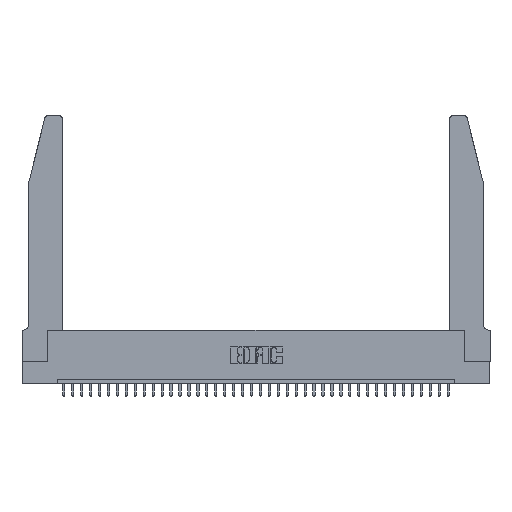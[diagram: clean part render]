
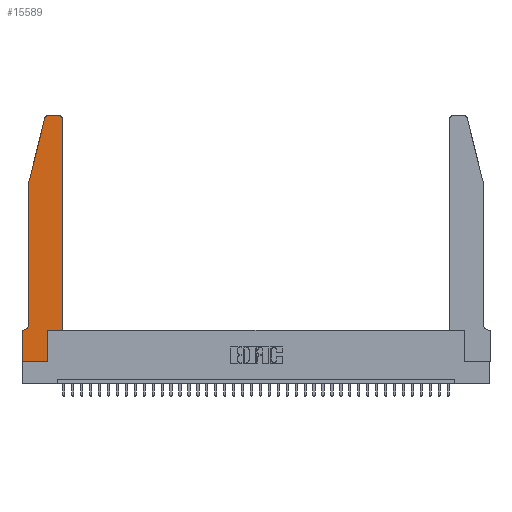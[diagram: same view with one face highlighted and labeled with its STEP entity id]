
A CAD part, top view. The second image highlights one B-rep face of the part: STEP entity #15589.
In plain terms, the highlighted planar face has unit normal (0, 0, 1).
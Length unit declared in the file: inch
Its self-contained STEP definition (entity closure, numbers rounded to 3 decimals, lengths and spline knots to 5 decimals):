
#540 = EDGE_CURVE ( 'NONE', #34609, #16465, #26308, .T. ) ;
#546 = CARTESIAN_POINT ( 'NONE',  ( 0.2605, 2.75, 0.37 ) ) ;
#603 = PLANE ( 'NONE',  #32592 ) ;
#1228 = CARTESIAN_POINT ( 'NONE',  ( 0.0755, 0.35, 0.37 ) ) ;
#1540 = VECTOR ( 'NONE', #35465, 39.37008 ) ;
#1619 = VERTEX_POINT ( 'NONE', #31086 ) ;
#1840 = ORIENTED_EDGE ( 'NONE', *, *, #20029, .T. ) ;
#1960 = CARTESIAN_POINT ( 'NONE',  ( 0.0055, 0.35, 0.37 ) ) ;
#1968 = CARTESIAN_POINT ( 'NONE',  ( 0.2865, 0.35, 0.37 ) ) ;
#2235 = DIRECTION ( 'NONE',  ( 1., 0., 0. ) ) ;
#3755 = CARTESIAN_POINT ( 'NONE',  ( 0.2865, 0.35, 0.37 ) ) ;
#3989 = CARTESIAN_POINT ( 'NONE',  ( 0.4205, 2.75, 0.37 ) ) ;
#4519 = CIRCLE ( 'NONE', #22841, 0.07 ) ;
#4787 = CIRCLE ( 'NONE', #18230, 0.03 ) ;
#5003 = DIRECTION ( 'NONE',  ( 1., 0., 0. ) ) ;
#5277 = VERTEX_POINT ( 'NONE', #36526 ) ;
#5345 = EDGE_CURVE ( 'NONE', #34705, #28668, #19008, .T. ) ;
#5517 = CARTESIAN_POINT ( 'NONE',  ( 0., 0.35, 0.37 ) ) ;
#5928 = DIRECTION ( 'NONE',  ( -1., 0., 0. ) ) ;
#6936 = CARTESIAN_POINT ( 'NONE',  ( 0.0755, 2., 0.37 ) ) ;
#7002 = LINE ( 'NONE', #23745, #1540 ) ;
#7393 = DIRECTION ( 'NONE',  ( -0.239, -0.971, 0. ) ) ;
#8667 = ORIENTED_EDGE ( 'NONE', *, *, #24339, .T. ) ;
#9014 = ORIENTED_EDGE ( 'NONE', *, *, #15074, .T. ) ;
#9318 = CARTESIAN_POINT ( 'NONE',  ( 0.284, 2.75, 0.37 ) ) ;
#9335 = VECTOR ( 'NONE', #25050, 39.37008 ) ;
#9835 = DIRECTION ( 'NONE',  ( 0., -1., 0. ) ) ;
#11094 = VERTEX_POINT ( 'NONE', #1960 ) ;
#11723 = DIRECTION ( 'NONE',  ( 0., 0., -1. ) ) ;
#12518 = AXIS2_PLACEMENT_3D ( 'NONE', #16449, #36681, #13529 ) ;
#13168 = CARTESIAN_POINT ( 'NONE',  ( 0., 0., 0.37 ) ) ;
#13414 = CARTESIAN_POINT ( 'NONE',  ( 0., 0., 0.37 ) ) ;
#13529 = DIRECTION ( 'NONE',  ( 1., 0., 0. ) ) ;
#14282 = CARTESIAN_POINT ( 'NONE',  ( 0.0055, 0.42, 0.37 ) ) ;
#14379 = EDGE_CURVE ( 'NONE', #15361, #34609, #24933, .T. ) ;
#15074 = EDGE_CURVE ( 'NONE', #36238, #25880, #33071, .T. ) ;
#15110 = EDGE_LOOP ( 'NONE', ( #33163, #36550, #19259, #37317, #23085, #8667, #28593, #1840, #9014, #28845, #21640, #17810 ) ) ;
#15361 = VERTEX_POINT ( 'NONE', #3989 ) ;
#15369 = VECTOR ( 'NONE', #26874, 39.37008 ) ;
#15589 = ADVANCED_FACE ( 'NONE', ( #24395 ), #603, .T. ) ;
#16449 = CARTESIAN_POINT ( 'NONE',  ( 0.284, 2.72, 0.37 ) ) ;
#16465 = VERTEX_POINT ( 'NONE', #19986 ) ;
#16531 = CARTESIAN_POINT ( 'NONE',  ( 0.4505, 0.35, 0.37 ) ) ;
#16654 = CARTESIAN_POINT ( 'NONE',  ( 0.0755, 2., 0.37 ) ) ;
#17066 = VECTOR ( 'NONE', #30768, 39.37008 ) ;
#17528 = CARTESIAN_POINT ( 'NONE',  ( 0.2865, 0., 0.37 ) ) ;
#17810 = ORIENTED_EDGE ( 'NONE', *, *, #17902, .T. ) ;
#17902 = EDGE_CURVE ( 'NONE', #27419, #15361, #4787, .T. ) ;
#17958 = LINE ( 'NONE', #16531, #9335 ) ;
#18153 = EDGE_CURVE ( 'NONE', #1619, #27419, #7002, .T. ) ;
#18230 = AXIS2_PLACEMENT_3D ( 'NONE', #37345, #22365, #5003 ) ;
#19008 = LINE ( 'NONE', #6936, #34515 ) ;
#19259 = ORIENTED_EDGE ( 'NONE', *, *, #28171, .T. ) ;
#19986 = CARTESIAN_POINT ( 'NONE',  ( 0.25487, 2.72718, 0.37 ) ) ;
#20029 = EDGE_CURVE ( 'NONE', #30661, #36238, #27767, .T. ) ;
#20062 = VECTOR ( 'NONE', #7393, 39.37008 ) ;
#20211 = LINE ( 'NONE', #13168, #17066 ) ;
#20534 = DIRECTION ( 'NONE',  ( 0., 0., 1. ) ) ;
#20587 = CARTESIAN_POINT ( 'NONE',  ( 0.4505, 2.72, 0.37 ) ) ;
#21640 = ORIENTED_EDGE ( 'NONE', *, *, #18153, .T. ) ;
#22273 = CARTESIAN_POINT ( 'NONE',  ( 0.0755, 0.42, 0.37 ) ) ;
#22365 = DIRECTION ( 'NONE',  ( 0., 0., 1. ) ) ;
#22668 = EDGE_CURVE ( 'NONE', #28668, #11094, #4519, .T. ) ;
#22841 = AXIS2_PLACEMENT_3D ( 'NONE', #14282, #11723, #5928 ) ;
#23085 = ORIENTED_EDGE ( 'NONE', *, *, #22668, .T. ) ;
#23745 = CARTESIAN_POINT ( 'NONE',  ( 0.4505, 0.35, 0.37 ) ) ;
#24071 = DIRECTION ( 'NONE',  ( 0., 1., 0. ) ) ;
#24339 = EDGE_CURVE ( 'NONE', #11094, #5277, #34871, .T. ) ;
#24395 = FACE_OUTER_BOUND ( 'NONE', #15110, .T. ) ;
#24608 = EDGE_CURVE ( 'NONE', #25880, #1619, #17958, .T. ) ;
#24933 = LINE ( 'NONE', #546, #15369 ) ;
#25050 = DIRECTION ( 'NONE',  ( 1., 0., 0. ) ) ;
#25880 = VERTEX_POINT ( 'NONE', #1968 ) ;
#25939 = VECTOR ( 'NONE', #2235, 39.37008 ) ;
#26308 = CIRCLE ( 'NONE', #12518, 0.03 ) ;
#26874 = DIRECTION ( 'NONE',  ( -1., 0., 0. ) ) ;
#27124 = VECTOR ( 'NONE', #36038, 39.37008 ) ;
#27419 = VERTEX_POINT ( 'NONE', #20587 ) ;
#27767 = LINE ( 'NONE', #13414, #25939 ) ;
#28171 = EDGE_CURVE ( 'NONE', #16465, #34705, #36558, .T. ) ;
#28593 = ORIENTED_EDGE ( 'NONE', *, *, #34353, .T. ) ;
#28668 = VERTEX_POINT ( 'NONE', #22273 ) ;
#28845 = ORIENTED_EDGE ( 'NONE', *, *, #24608, .T. ) ;
#29255 = CARTESIAN_POINT ( 'NONE',  ( 0., 0., 0.37 ) ) ;
#29479 = DIRECTION ( 'NONE',  ( 1., 0., 0. ) ) ;
#30661 = VERTEX_POINT ( 'NONE', #29255 ) ;
#30768 = DIRECTION ( 'NONE',  ( 0., -1., 0. ) ) ;
#31086 = CARTESIAN_POINT ( 'NONE',  ( 0.4505, 0.35, 0.37 ) ) ;
#32592 = AXIS2_PLACEMENT_3D ( 'NONE', #5517, #20534, #29479 ) ;
#32731 = CARTESIAN_POINT ( 'NONE',  ( 0.0755, 2., 0.37 ) ) ;
#33071 = LINE ( 'NONE', #3755, #34472 ) ;
#33163 = ORIENTED_EDGE ( 'NONE', *, *, #14379, .T. ) ;
#34353 = EDGE_CURVE ( 'NONE', #5277, #30661, #20211, .T. ) ;
#34472 = VECTOR ( 'NONE', #24071, 39.37008 ) ;
#34515 = VECTOR ( 'NONE', #9835, 39.37008 ) ;
#34609 = VERTEX_POINT ( 'NONE', #9318 ) ;
#34705 = VERTEX_POINT ( 'NONE', #32731 ) ;
#34871 = LINE ( 'NONE', #1228, #27124 ) ;
#35465 = DIRECTION ( 'NONE',  ( 0., 1., 0. ) ) ;
#36038 = DIRECTION ( 'NONE',  ( -1., 0., 0. ) ) ;
#36238 = VERTEX_POINT ( 'NONE', #17528 ) ;
#36526 = CARTESIAN_POINT ( 'NONE',  ( 0., 0.35, 0.37 ) ) ;
#36550 = ORIENTED_EDGE ( 'NONE', *, *, #540, .T. ) ;
#36558 = LINE ( 'NONE', #16654, #20062 ) ;
#36681 = DIRECTION ( 'NONE',  ( 0., 0., 1. ) ) ;
#37317 = ORIENTED_EDGE ( 'NONE', *, *, #5345, .T. ) ;
#37345 = CARTESIAN_POINT ( 'NONE',  ( 0.4205, 2.72, 0.37 ) ) ;
